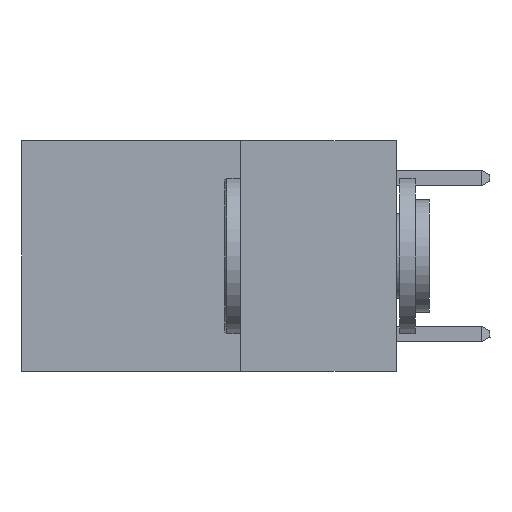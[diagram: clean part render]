
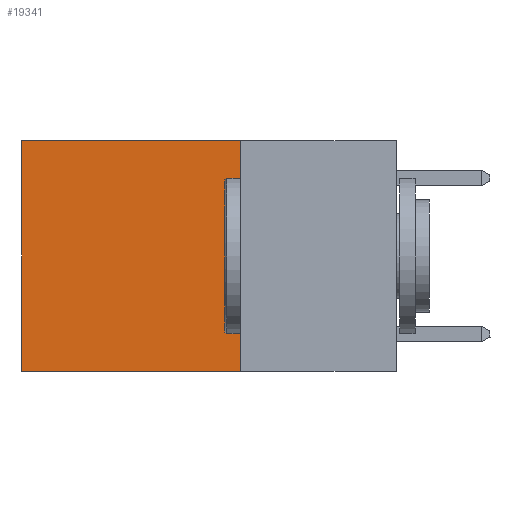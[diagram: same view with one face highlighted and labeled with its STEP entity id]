
A CAD part, left-side view. The second image highlights one B-rep face of the part: STEP entity #19341.
In plain terms, the highlighted planar face has unit normal (-1, 0, 0).
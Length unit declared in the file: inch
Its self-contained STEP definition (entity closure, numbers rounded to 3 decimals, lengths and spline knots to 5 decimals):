
#53 = FACE_OUTER_BOUND ( 'NONE', #1089, .T. ) ;
#476 = CARTESIAN_POINT ( 'NONE',  ( 0.2625, 0.6, -0.37 ) ) ;
#1089 = EDGE_LOOP ( 'NONE', ( #9579, #4196, #7780, #16830 ) ) ;
#1699 = VECTOR ( 'NONE', #14991, 39.37008 ) ;
#2037 = LINE ( 'NONE', #15018, #1699 ) ;
#2042 = LINE ( 'NONE', #17127, #6204 ) ;
#2812 = EDGE_CURVE ( 'NONE', #17719, #5388, #2037, .T. ) ;
#3340 = CARTESIAN_POINT ( 'NONE',  ( 0.2625, 0.25, -0.37 ) ) ;
#4196 = ORIENTED_EDGE ( 'NONE', *, *, #20757, .F. ) ;
#4359 = CARTESIAN_POINT ( 'NONE',  ( 0.2625, 0.6, 0. ) ) ;
#5167 = CARTESIAN_POINT ( 'NONE',  ( 0.2625, 0.25, 0. ) ) ;
#5300 = DIRECTION ( 'NONE',  ( 0., 1., 0. ) ) ;
#5388 = VERTEX_POINT ( 'NONE', #476 ) ;
#5542 = PLANE ( 'NONE',  #19794 ) ;
#6204 = VECTOR ( 'NONE', #5300, 39.37008 ) ;
#6699 = EDGE_CURVE ( 'NONE', #20088, #10911, #15338, .T. ) ;
#7301 = DIRECTION ( 'NONE',  ( 1., 0., 0. ) ) ;
#7780 = ORIENTED_EDGE ( 'NONE', *, *, #6699, .F. ) ;
#8329 = CARTESIAN_POINT ( 'NONE',  ( 0.2625, 0.25, 0. ) ) ;
#9568 = CARTESIAN_POINT ( 'NONE',  ( 0.2625, 0.25, 0. ) ) ;
#9579 = ORIENTED_EDGE ( 'NONE', *, *, #2812, .T. ) ;
#10002 = DIRECTION ( 'NONE',  ( 0., 1., 0. ) ) ;
#10911 = VERTEX_POINT ( 'NONE', #3340 ) ;
#11440 = EDGE_CURVE ( 'NONE', #20088, #17719, #14340, .T. ) ;
#13040 = DIRECTION ( 'NONE',  ( 0., 0., -1. ) ) ;
#14294 = VECTOR ( 'NONE', #10002, 39.37008 ) ;
#14340 = LINE ( 'NONE', #8329, #14294 ) ;
#14991 = DIRECTION ( 'NONE',  ( 0., 0., -1. ) ) ;
#15018 = CARTESIAN_POINT ( 'NONE',  ( 0.2625, 0.6, 0. ) ) ;
#15231 = VECTOR ( 'NONE', #13040, 39.37008 ) ;
#15338 = LINE ( 'NONE', #9568, #15231 ) ;
#16830 = ORIENTED_EDGE ( 'NONE', *, *, #11440, .T. ) ;
#17127 = CARTESIAN_POINT ( 'NONE',  ( 0.2625, 0.25, -0.37 ) ) ;
#17361 = CARTESIAN_POINT ( 'NONE',  ( 0.2625, 0.25, 0. ) ) ;
#17719 = VERTEX_POINT ( 'NONE', #4359 ) ;
#18943 = DIRECTION ( 'NONE',  ( 0., 0., -1. ) ) ;
#19341 = ADVANCED_FACE ( 'NONE', ( #53 ), #5542, .F. ) ;
#19794 = AXIS2_PLACEMENT_3D ( 'NONE', #17361, #7301, #18943 ) ;
#20088 = VERTEX_POINT ( 'NONE', #5167 ) ;
#20757 = EDGE_CURVE ( 'NONE', #10911, #5388, #2042, .T. ) ;
